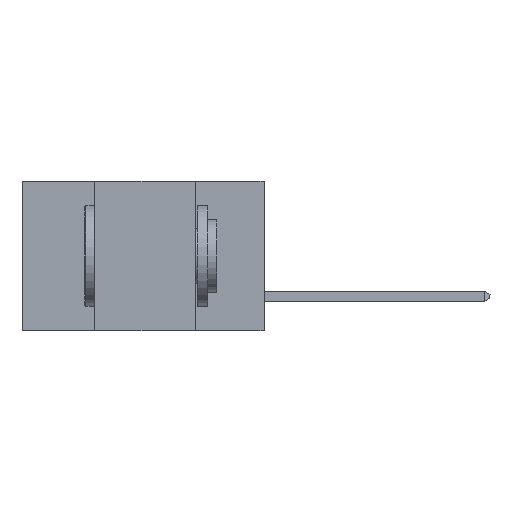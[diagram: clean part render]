
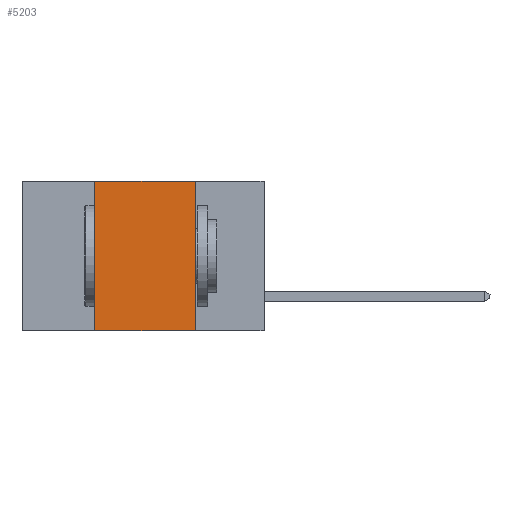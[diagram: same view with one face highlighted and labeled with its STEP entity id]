
A CAD part, left-side view. The second image highlights one B-rep face of the part: STEP entity #5203.
In plain terms, the highlighted planar face has unit normal (-1, 0, 0).
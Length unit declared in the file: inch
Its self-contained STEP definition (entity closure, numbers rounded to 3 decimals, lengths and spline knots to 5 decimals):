
#54 = VECTOR ( 'NONE', #7412, 39.37008 ) ;
#120 = ORIENTED_EDGE ( 'NONE', *, *, #4723, .F. ) ;
#206 = CARTESIAN_POINT ( 'NONE',  ( 0., 0.6, -0.37 ) ) ;
#568 = AXIS2_PLACEMENT_3D ( 'NONE', #9952, #4523, #8409 ) ;
#605 = EDGE_CURVE ( 'NONE', #4641, #1125, #7566, .T. ) ;
#831 = VERTEX_POINT ( 'NONE', #8857 ) ;
#1125 = VERTEX_POINT ( 'NONE', #7452 ) ;
#1221 = LINE ( 'NONE', #4325, #6138 ) ;
#1861 = VERTEX_POINT ( 'NONE', #3117 ) ;
#2172 = VECTOR ( 'NONE', #6826, 39.37008 ) ;
#2188 = EDGE_CURVE ( 'NONE', #1125, #1861, #1221, .T. ) ;
#2801 = CARTESIAN_POINT ( 'NONE',  ( 0., 0.17, -0.37 ) ) ;
#2975 = ORIENTED_EDGE ( 'NONE', *, *, #3311, .T. ) ;
#3003 = ORIENTED_EDGE ( 'NONE', *, *, #605, .F. ) ;
#3117 = CARTESIAN_POINT ( 'NONE',  ( 0., 0.17, 0. ) ) ;
#3311 = EDGE_CURVE ( 'NONE', #4641, #831, #8169, .T. ) ;
#4325 = CARTESIAN_POINT ( 'NONE',  ( 0., 0.6, 0. ) ) ;
#4523 = DIRECTION ( 'NONE',  ( 1., 0., 0. ) ) ;
#4641 = VERTEX_POINT ( 'NONE', #5686 ) ;
#4723 = EDGE_CURVE ( 'NONE', #1861, #831, #5111, .T. ) ;
#5111 = LINE ( 'NONE', #2801, #2172 ) ;
#5203 = ADVANCED_FACE ( 'NONE', ( #9913 ), #5242, .F. ) ;
#5242 = PLANE ( 'NONE',  #568 ) ;
#5686 = CARTESIAN_POINT ( 'NONE',  ( 0., 0.42, -0.37 ) ) ;
#6138 = VECTOR ( 'NONE', #7430, 39.37008 ) ;
#6226 = VECTOR ( 'NONE', #8850, 39.37008 ) ;
#6826 = DIRECTION ( 'NONE',  ( 0., 0., -1. ) ) ;
#7412 = DIRECTION ( 'NONE',  ( 0., 0., 1. ) ) ;
#7430 = DIRECTION ( 'NONE',  ( 0., -1., 0. ) ) ;
#7452 = CARTESIAN_POINT ( 'NONE',  ( 0., 0.42, 0. ) ) ;
#7566 = LINE ( 'NONE', #9828, #54 ) ;
#8169 = LINE ( 'NONE', #206, #6226 ) ;
#8409 = DIRECTION ( 'NONE',  ( 0., 0., -1. ) ) ;
#8434 = EDGE_LOOP ( 'NONE', ( #120, #9293, #3003, #2975 ) ) ;
#8850 = DIRECTION ( 'NONE',  ( 0., -1., 0. ) ) ;
#8857 = CARTESIAN_POINT ( 'NONE',  ( 0., 0.17, -0.37 ) ) ;
#9293 = ORIENTED_EDGE ( 'NONE', *, *, #2188, .F. ) ;
#9828 = CARTESIAN_POINT ( 'NONE',  ( 0., 0.42, -0.37 ) ) ;
#9913 = FACE_OUTER_BOUND ( 'NONE', #8434, .T. ) ;
#9952 = CARTESIAN_POINT ( 'NONE',  ( 0., 0.6, 0. ) ) ;
